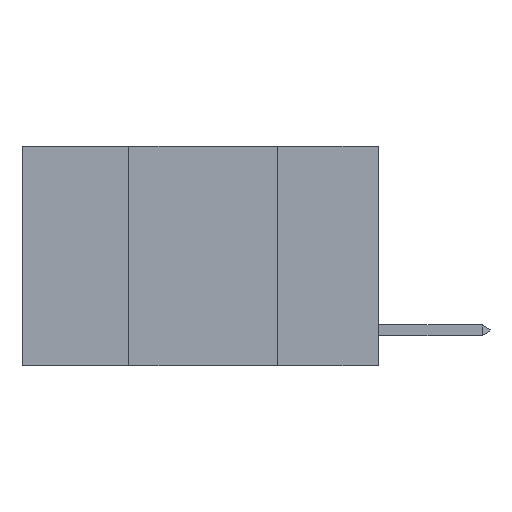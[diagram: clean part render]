
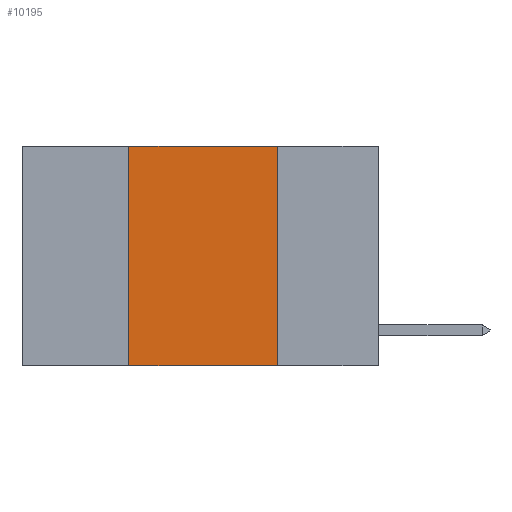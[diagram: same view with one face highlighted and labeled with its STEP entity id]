
A CAD part, left-side view. The second image highlights one B-rep face of the part: STEP entity #10195.
In plain terms, the highlighted planar face has unit normal (-1, 0, 0).
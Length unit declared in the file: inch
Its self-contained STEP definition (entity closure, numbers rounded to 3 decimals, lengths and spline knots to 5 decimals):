
#833 = EDGE_LOOP ( 'NONE', ( #23415, #6736, #5807, #22250 ) ) ;
#848 = CARTESIAN_POINT ( 'NONE',  ( 0., 0.17, 0. ) ) ;
#1320 = CARTESIAN_POINT ( 'NONE',  ( 0., 0.6, 0. ) ) ;
#2965 = CARTESIAN_POINT ( 'NONE',  ( 0., 0.42, 0. ) ) ;
#3102 = DIRECTION ( 'NONE',  ( 0., 0., -1. ) ) ;
#3514 = LINE ( 'NONE', #6184, #14480 ) ;
#3960 = DIRECTION ( 'NONE',  ( 0., 0., 1. ) ) ;
#4391 = VERTEX_POINT ( 'NONE', #2965 ) ;
#4440 = CARTESIAN_POINT ( 'NONE',  ( 0., 0.17, 0. ) ) ;
#5297 = VERTEX_POINT ( 'NONE', #6981 ) ;
#5807 = ORIENTED_EDGE ( 'NONE', *, *, #24627, .F. ) ;
#6184 = CARTESIAN_POINT ( 'NONE',  ( 0., 0.42, 0. ) ) ;
#6599 = EDGE_CURVE ( 'NONE', #14415, #5297, #8313, .T. ) ;
#6736 = ORIENTED_EDGE ( 'NONE', *, *, #27010, .F. ) ;
#6981 = CARTESIAN_POINT ( 'NONE',  ( 0., 0.17, -0.37 ) ) ;
#7209 = CARTESIAN_POINT ( 'NONE',  ( 0., 0.6, -0.37 ) ) ;
#7805 = CARTESIAN_POINT ( 'NONE',  ( 0., 0.6, 0. ) ) ;
#8313 = LINE ( 'NONE', #7209, #19210 ) ;
#8562 = CARTESIAN_POINT ( 'NONE',  ( 0., 0.42, -0.37 ) ) ;
#10001 = DIRECTION ( 'NONE',  ( 1., 0., 0. ) ) ;
#10084 = EDGE_CURVE ( 'NONE', #18037, #5297, #10150, .T. ) ;
#10150 = LINE ( 'NONE', #848, #21017 ) ;
#10195 = ADVANCED_FACE ( 'NONE', ( #24047 ), #20836, .F. ) ;
#13989 = VECTOR ( 'NONE', #18840, 39.37008 ) ;
#14415 = VERTEX_POINT ( 'NONE', #8562 ) ;
#14480 = VECTOR ( 'NONE', #3960, 39.37008 ) ;
#16037 = AXIS2_PLACEMENT_3D ( 'NONE', #7805, #10001, #25192 ) ;
#18037 = VERTEX_POINT ( 'NONE', #4440 ) ;
#18840 = DIRECTION ( 'NONE',  ( 0., -1., 0. ) ) ;
#19210 = VECTOR ( 'NONE', #20256, 39.37008 ) ;
#20256 = DIRECTION ( 'NONE',  ( 0., -1., 0. ) ) ;
#20836 = PLANE ( 'NONE',  #16037 ) ;
#21017 = VECTOR ( 'NONE', #3102, 39.37008 ) ;
#22250 = ORIENTED_EDGE ( 'NONE', *, *, #6599, .T. ) ;
#23415 = ORIENTED_EDGE ( 'NONE', *, *, #10084, .F. ) ;
#24047 = FACE_OUTER_BOUND ( 'NONE', #833, .T. ) ;
#24627 = EDGE_CURVE ( 'NONE', #14415, #4391, #3514, .T. ) ;
#24831 = LINE ( 'NONE', #1320, #13989 ) ;
#25192 = DIRECTION ( 'NONE',  ( 0., 0., -1. ) ) ;
#27010 = EDGE_CURVE ( 'NONE', #4391, #18037, #24831, .T. ) ;
